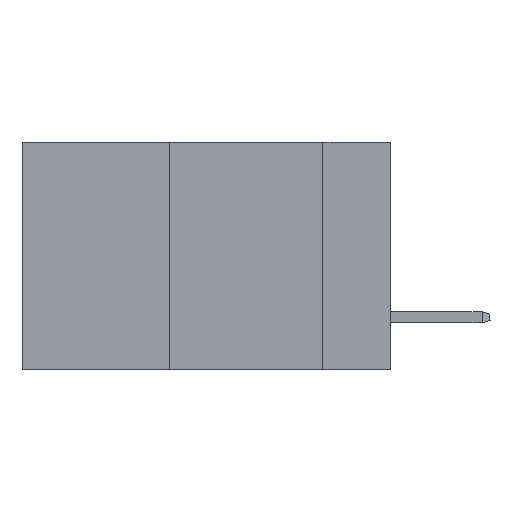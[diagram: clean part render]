
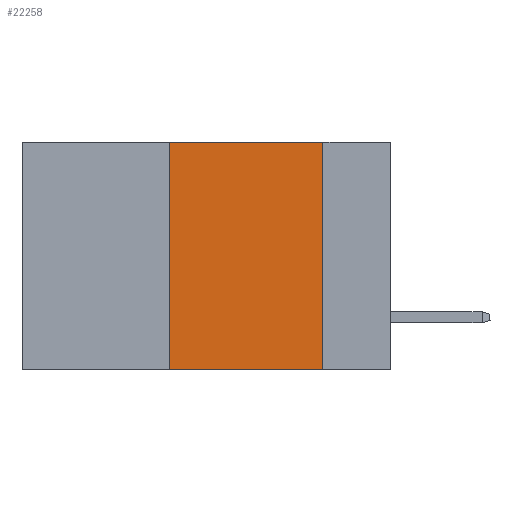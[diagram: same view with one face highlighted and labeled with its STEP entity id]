
A CAD part, left-side view. The second image highlights one B-rep face of the part: STEP entity #22258.
In plain terms, the highlighted planar face has unit normal (-1, 0, 0).
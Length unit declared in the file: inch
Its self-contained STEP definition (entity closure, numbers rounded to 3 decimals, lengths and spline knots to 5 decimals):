
#520 = EDGE_CURVE ( 'NONE', #7638, #19871, #10904, .T. ) ;
#673 = DIRECTION ( 'NONE',  ( 0., 0., 1. ) ) ;
#2153 = FACE_OUTER_BOUND ( 'NONE', #18720, .T. ) ;
#2665 = VECTOR ( 'NONE', #673, 39.37008 ) ;
#3570 = AXIS2_PLACEMENT_3D ( 'NONE', #20443, #27431, #25053 ) ;
#4474 = CARTESIAN_POINT ( 'NONE',  ( 0., 0.11, 0. ) ) ;
#6058 = VECTOR ( 'NONE', #26387, 39.37008 ) ;
#6285 = PLANE ( 'NONE',  #3570 ) ;
#6830 = DIRECTION ( 'NONE',  ( 0., -1., 0. ) ) ;
#7315 = CARTESIAN_POINT ( 'NONE',  ( 0., 0.6, -0.37 ) ) ;
#7638 = VERTEX_POINT ( 'NONE', #12821 ) ;
#7640 = CARTESIAN_POINT ( 'NONE',  ( 0., 0.11, -0.37 ) ) ;
#8109 = EDGE_CURVE ( 'NONE', #29525, #19871, #27089, .T. ) ;
#8208 = EDGE_CURVE ( 'NONE', #17647, #7638, #17526, .T. ) ;
#10904 = LINE ( 'NONE', #4474, #21631 ) ;
#11631 = VECTOR ( 'NONE', #6830, 39.37008 ) ;
#12821 = CARTESIAN_POINT ( 'NONE',  ( 0., 0.11, 0. ) ) ;
#14462 = ORIENTED_EDGE ( 'NONE', *, *, #520, .F. ) ;
#14487 = LINE ( 'NONE', #14831, #2665 ) ;
#14831 = CARTESIAN_POINT ( 'NONE',  ( 0., 0.36, 0. ) ) ;
#16216 = DIRECTION ( 'NONE',  ( 0., 0., -1. ) ) ;
#17526 = LINE ( 'NONE', #20977, #11631 ) ;
#17647 = VERTEX_POINT ( 'NONE', #19984 ) ;
#18720 = EDGE_LOOP ( 'NONE', ( #14462, #29489, #20645, #29389 ) ) ;
#19871 = VERTEX_POINT ( 'NONE', #7640 ) ;
#19984 = CARTESIAN_POINT ( 'NONE',  ( 0., 0.36, 0. ) ) ;
#20443 = CARTESIAN_POINT ( 'NONE',  ( 0., 0.6, 0. ) ) ;
#20645 = ORIENTED_EDGE ( 'NONE', *, *, #23175, .F. ) ;
#20977 = CARTESIAN_POINT ( 'NONE',  ( 0., 0.6, 0. ) ) ;
#21631 = VECTOR ( 'NONE', #16216, 39.37008 ) ;
#22258 = ADVANCED_FACE ( 'NONE', ( #2153 ), #6285, .F. ) ;
#23175 = EDGE_CURVE ( 'NONE', #29525, #17647, #14487, .T. ) ;
#25053 = DIRECTION ( 'NONE',  ( 0., 0., -1. ) ) ;
#26387 = DIRECTION ( 'NONE',  ( 0., -1., 0. ) ) ;
#26697 = CARTESIAN_POINT ( 'NONE',  ( 0., 0.36, -0.37 ) ) ;
#27089 = LINE ( 'NONE', #7315, #6058 ) ;
#27431 = DIRECTION ( 'NONE',  ( 1., 0., 0. ) ) ;
#29389 = ORIENTED_EDGE ( 'NONE', *, *, #8109, .T. ) ;
#29489 = ORIENTED_EDGE ( 'NONE', *, *, #8208, .F. ) ;
#29525 = VERTEX_POINT ( 'NONE', #26697 ) ;
